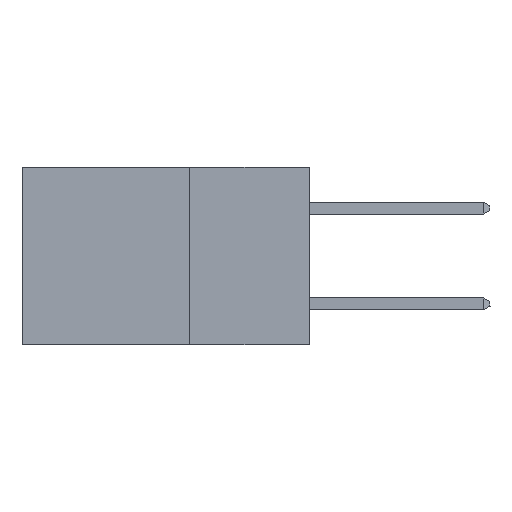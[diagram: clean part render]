
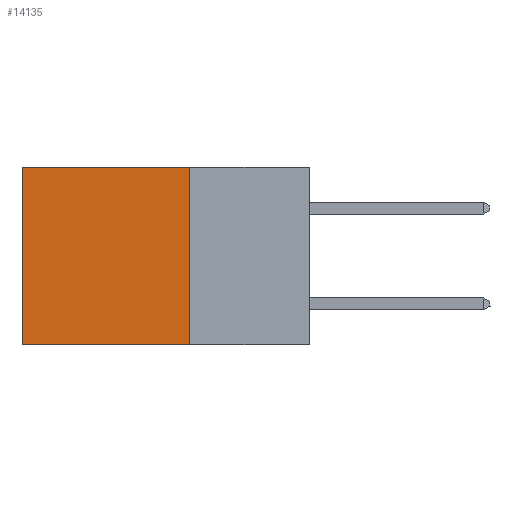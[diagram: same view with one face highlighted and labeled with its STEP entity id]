
A CAD part, left-side view. The second image highlights one B-rep face of the part: STEP entity #14135.
In plain terms, the highlighted planar face has unit normal (-1, 0, 0).
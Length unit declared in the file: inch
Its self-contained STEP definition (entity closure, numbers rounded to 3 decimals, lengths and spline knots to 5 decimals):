
#1270 = CARTESIAN_POINT ( 'NONE',  ( 0.2875, 0.25, -0.37 ) ) ;
#1387 = VECTOR ( 'NONE', #3792, 39.37008 ) ;
#1393 = CARTESIAN_POINT ( 'NONE',  ( 0.2875, 0.6, -0.37 ) ) ;
#2549 = AXIS2_PLACEMENT_3D ( 'NONE', #14267, #8890, #28151 ) ;
#3050 = ORIENTED_EDGE ( 'NONE', *, *, #31662, .F. ) ;
#3792 = DIRECTION ( 'NONE',  ( 0., 0., -1. ) ) ;
#5334 = VERTEX_POINT ( 'NONE', #6346 ) ;
#6346 = CARTESIAN_POINT ( 'NONE',  ( 0.2875, 0.25, -0.37 ) ) ;
#6886 = VERTEX_POINT ( 'NONE', #12068 ) ;
#8483 = ORIENTED_EDGE ( 'NONE', *, *, #14166, .T. ) ;
#8890 = DIRECTION ( 'NONE',  ( 1., 0., 0. ) ) ;
#11522 = LINE ( 'NONE', #1270, #24905 ) ;
#11996 = ORIENTED_EDGE ( 'NONE', *, *, #22884, .F. ) ;
#12068 = CARTESIAN_POINT ( 'NONE',  ( 0.2875, 0.6, 0. ) ) ;
#12641 = EDGE_LOOP ( 'NONE', ( #20373, #3050, #11996, #8483 ) ) ;
#14135 = ADVANCED_FACE ( 'NONE', ( #33754 ), #25720, .F. ) ;
#14166 = EDGE_CURVE ( 'NONE', #19269, #6886, #28590, .T. ) ;
#14267 = CARTESIAN_POINT ( 'NONE',  ( 0.2875, 0.25, 0. ) ) ;
#15071 = LINE ( 'NONE', #22180, #1387 ) ;
#19269 = VERTEX_POINT ( 'NONE', #19588 ) ;
#19588 = CARTESIAN_POINT ( 'NONE',  ( 0.2875, 0.25, 0. ) ) ;
#20373 = ORIENTED_EDGE ( 'NONE', *, *, #33852, .T. ) ;
#21267 = LINE ( 'NONE', #33046, #32483 ) ;
#21964 = DIRECTION ( 'NONE',  ( 0., 0., -1. ) ) ;
#22180 = CARTESIAN_POINT ( 'NONE',  ( 0.2875, 0.25, 0. ) ) ;
#22884 = EDGE_CURVE ( 'NONE', #19269, #5334, #15071, .T. ) ;
#24905 = VECTOR ( 'NONE', #31050, 39.37008 ) ;
#25113 = VECTOR ( 'NONE', #30774, 39.37008 ) ;
#25720 = PLANE ( 'NONE',  #2549 ) ;
#28151 = DIRECTION ( 'NONE',  ( 0., 0., -1. ) ) ;
#28590 = LINE ( 'NONE', #30884, #25113 ) ;
#30774 = DIRECTION ( 'NONE',  ( 0., 1., 0. ) ) ;
#30884 = CARTESIAN_POINT ( 'NONE',  ( 0.2875, 0.25, 0. ) ) ;
#31050 = DIRECTION ( 'NONE',  ( 0., 1., 0. ) ) ;
#31662 = EDGE_CURVE ( 'NONE', #5334, #31699, #11522, .T. ) ;
#31699 = VERTEX_POINT ( 'NONE', #1393 ) ;
#32483 = VECTOR ( 'NONE', #21964, 39.37008 ) ;
#33046 = CARTESIAN_POINT ( 'NONE',  ( 0.2875, 0.6, 0. ) ) ;
#33754 = FACE_OUTER_BOUND ( 'NONE', #12641, .T. ) ;
#33852 = EDGE_CURVE ( 'NONE', #6886, #31699, #21267, .T. ) ;
